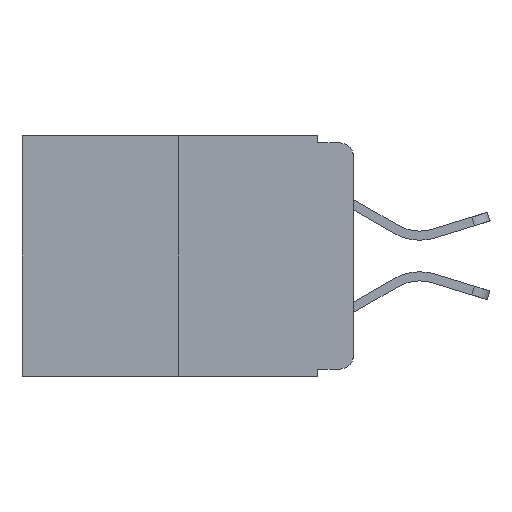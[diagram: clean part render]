
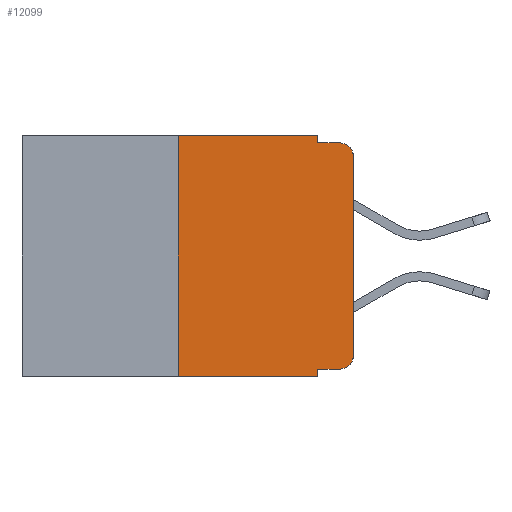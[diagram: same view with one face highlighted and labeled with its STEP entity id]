
A CAD part, left-side view. The second image highlights one B-rep face of the part: STEP entity #12099.
In plain terms, the highlighted planar face has unit normal (-1, 0, 0).
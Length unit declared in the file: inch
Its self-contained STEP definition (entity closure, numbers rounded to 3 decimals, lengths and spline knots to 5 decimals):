
#166 = CARTESIAN_POINT ( 'NONE',  ( 0., 0.473, -0.343 ) ) ;
#280 = EDGE_CURVE ( 'NONE', #3989, #8716, #11203, .T. ) ;
#537 = ORIENTED_EDGE ( 'NONE', *, *, #11369, .F. ) ;
#553 = ORIENTED_EDGE ( 'NONE', *, *, #280, .F. ) ;
#554 = VERTEX_POINT ( 'NONE', #7914 ) ;
#859 = DIRECTION ( 'NONE',  ( 0., 0., -1. ) ) ;
#992 = LINE ( 'NONE', #166, #11081 ) ;
#1020 = EDGE_CURVE ( 'NONE', #2629, #5043, #7951, .T. ) ;
#1467 = CARTESIAN_POINT ( 'NONE',  ( 0., 0.051, -0.01 ) ) ;
#1742 = DIRECTION ( 'NONE',  ( -1., 0., 0. ) ) ;
#2055 = CIRCLE ( 'NONE', #2889, 0.02 ) ;
#2075 = ORIENTED_EDGE ( 'NONE', *, *, #10133, .T. ) ;
#2629 = VERTEX_POINT ( 'NONE', #7915 ) ;
#2746 = CARTESIAN_POINT ( 'NONE',  ( 0., 0.02, -0.03 ) ) ;
#2889 = AXIS2_PLACEMENT_3D ( 'NONE', #4394, #1742, #859 ) ;
#3200 = EDGE_CURVE ( 'NONE', #2629, #4461, #3749, .T. ) ;
#3363 = CARTESIAN_POINT ( 'NONE',  ( 0., 0.051, 0. ) ) ;
#3429 = ORIENTED_EDGE ( 'NONE', *, *, #5130, .T. ) ;
#3749 = LINE ( 'NONE', #4284, #7134 ) ;
#3836 = DIRECTION ( 'NONE',  ( 0., 0., -1. ) ) ;
#3907 = EDGE_CURVE ( 'NONE', #4461, #7858, #2055, .T. ) ;
#3989 = VERTEX_POINT ( 'NONE', #4136 ) ;
#4037 = CARTESIAN_POINT ( 'NONE',  ( 0., 0.051, 0. ) ) ;
#4136 = CARTESIAN_POINT ( 'NONE',  ( 0., 0.25, -0.343 ) ) ;
#4223 = PLANE ( 'NONE',  #11176 ) ;
#4275 = DIRECTION ( 'NONE',  ( 0., -1., 0. ) ) ;
#4284 = CARTESIAN_POINT ( 'NONE',  ( 0., 0.051, -0.333 ) ) ;
#4394 = CARTESIAN_POINT ( 'NONE',  ( 0., 0.02, -0.313 ) ) ;
#4411 = EDGE_CURVE ( 'NONE', #8716, #6978, #7099, .T. ) ;
#4461 = VERTEX_POINT ( 'NONE', #11428 ) ;
#4551 = VERTEX_POINT ( 'NONE', #4724 ) ;
#4724 = CARTESIAN_POINT ( 'NONE',  ( 0., 0., -0.03 ) ) ;
#4790 = DIRECTION ( 'NONE',  ( 0., 0., -1. ) ) ;
#4880 = ORIENTED_EDGE ( 'NONE', *, *, #10763, .T. ) ;
#5043 = VERTEX_POINT ( 'NONE', #9207 ) ;
#5099 = DIRECTION ( 'NONE',  ( 0., 0., -1. ) ) ;
#5130 = EDGE_CURVE ( 'NONE', #3989, #5043, #992, .T. ) ;
#5300 = CARTESIAN_POINT ( 'NONE',  ( 0., 0.473, 0. ) ) ;
#6117 = VECTOR ( 'NONE', #10127, 39.37008 ) ;
#6340 = DIRECTION ( 'NONE',  ( 1., 0., 0. ) ) ;
#6499 = VECTOR ( 'NONE', #5099, 39.37008 ) ;
#6978 = VERTEX_POINT ( 'NONE', #7046 ) ;
#7046 = CARTESIAN_POINT ( 'NONE',  ( 0., 0.051, 0. ) ) ;
#7099 = LINE ( 'NONE', #8165, #11822 ) ;
#7134 = VECTOR ( 'NONE', #4275, 39.37008 ) ;
#7136 = ORIENTED_EDGE ( 'NONE', *, *, #12617, .F. ) ;
#7142 = CIRCLE ( 'NONE', #11247, 0.02 ) ;
#7276 = VECTOR ( 'NONE', #10516, 39.37008 ) ;
#7431 = ORIENTED_EDGE ( 'NONE', *, *, #4411, .F. ) ;
#7475 = CARTESIAN_POINT ( 'NONE',  ( 0., 0., -0.313 ) ) ;
#7640 = VECTOR ( 'NONE', #4790, 39.37008 ) ;
#7858 = VERTEX_POINT ( 'NONE', #7475 ) ;
#7914 = CARTESIAN_POINT ( 'NONE',  ( 0., 0.051, -0.01 ) ) ;
#7915 = CARTESIAN_POINT ( 'NONE',  ( 0., 0.051, -0.333 ) ) ;
#7951 = LINE ( 'NONE', #3363, #7640 ) ;
#8165 = CARTESIAN_POINT ( 'NONE',  ( 0., 0.473, 0. ) ) ;
#8205 = ORIENTED_EDGE ( 'NONE', *, *, #3200, .T. ) ;
#8405 = DIRECTION ( 'NONE',  ( 0., -1., 0. ) ) ;
#8677 = DIRECTION ( 'NONE',  ( 0., -1., 0. ) ) ;
#8716 = VERTEX_POINT ( 'NONE', #11178 ) ;
#8968 = DIRECTION ( 'NONE',  ( 0., 0., 1. ) ) ;
#9207 = CARTESIAN_POINT ( 'NONE',  ( 0., 0.051, -0.343 ) ) ;
#9784 = DIRECTION ( 'NONE',  ( -1., 0., 0. ) ) ;
#9928 = CARTESIAN_POINT ( 'NONE',  ( 0., 0., 0. ) ) ;
#9952 = CARTESIAN_POINT ( 'NONE',  ( 0., 0.25, 0. ) ) ;
#9966 = FACE_OUTER_BOUND ( 'NONE', #11350, .T. ) ;
#10127 = DIRECTION ( 'NONE',  ( 0., 0., 1. ) ) ;
#10133 = EDGE_CURVE ( 'NONE', #7858, #4551, #10278, .T. ) ;
#10278 = LINE ( 'NONE', #9928, #12444 ) ;
#10402 = LINE ( 'NONE', #1467, #7276 ) ;
#10516 = DIRECTION ( 'NONE',  ( 0., -1., 0. ) ) ;
#10763 = EDGE_CURVE ( 'NONE', #4551, #12682, #7142, .T. ) ;
#11081 = VECTOR ( 'NONE', #8677, 39.37008 ) ;
#11176 = AXIS2_PLACEMENT_3D ( 'NONE', #5300, #6340, #12930 ) ;
#11178 = CARTESIAN_POINT ( 'NONE',  ( 0., 0.25, 0. ) ) ;
#11203 = LINE ( 'NONE', #9952, #6117 ) ;
#11247 = AXIS2_PLACEMENT_3D ( 'NONE', #2746, #9784, #3836 ) ;
#11350 = EDGE_LOOP ( 'NONE', ( #2075, #4880, #537, #7136, #7431, #553, #3429, #12148, #8205, #11584 ) ) ;
#11369 = EDGE_CURVE ( 'NONE', #554, #12682, #10402, .T. ) ;
#11428 = CARTESIAN_POINT ( 'NONE',  ( 0., 0.02, -0.333 ) ) ;
#11584 = ORIENTED_EDGE ( 'NONE', *, *, #3907, .T. ) ;
#11822 = VECTOR ( 'NONE', #8405, 39.37008 ) ;
#11842 = LINE ( 'NONE', #4037, #6499 ) ;
#12099 = ADVANCED_FACE ( 'NONE', ( #9966 ), #4223, .F. ) ;
#12148 = ORIENTED_EDGE ( 'NONE', *, *, #1020, .F. ) ;
#12444 = VECTOR ( 'NONE', #8968, 39.37008 ) ;
#12617 = EDGE_CURVE ( 'NONE', #6978, #554, #11842, .T. ) ;
#12682 = VERTEX_POINT ( 'NONE', #12815 ) ;
#12815 = CARTESIAN_POINT ( 'NONE',  ( 0., 0.02, -0.01 ) ) ;
#12930 = DIRECTION ( 'NONE',  ( 0., 0., -1. ) ) ;
